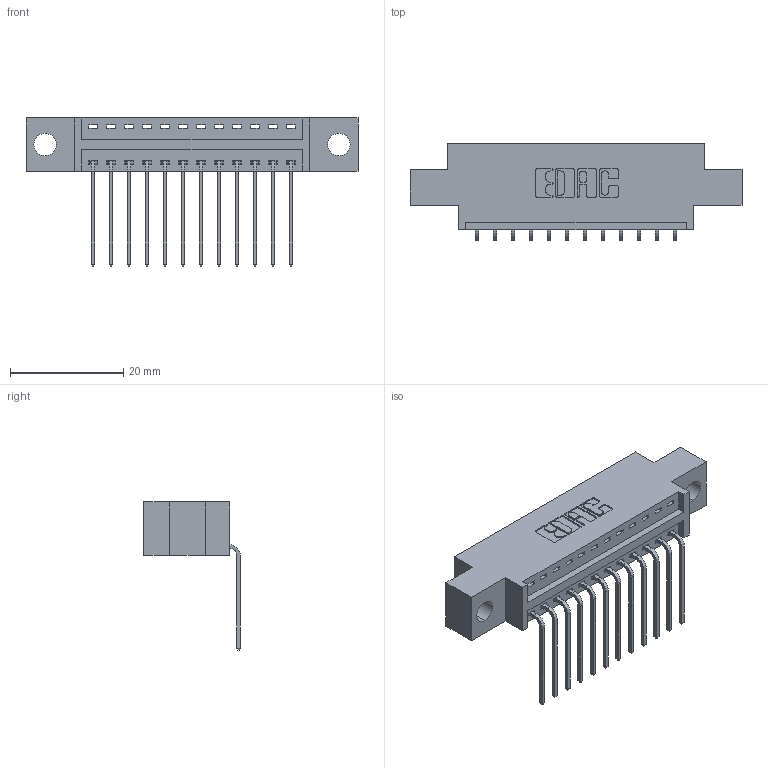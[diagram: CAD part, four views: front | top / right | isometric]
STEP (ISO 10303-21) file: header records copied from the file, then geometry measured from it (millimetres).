
FILE_DESCRIPTION (( 'STEP AP203' ), '1' );
FILE_NAME ('346-012-559-604.STEP', '2022-05-05T03:38:17', ( '' ), ( '' ), 'SwSTEP 2.0', 'SolidWorks 2020', '' );
FILE_SCHEMA (( 'CONFIG_CONTROL_DESIGN' ));
Length unit declared in the file: inch
Products named in the file (3): 345-292-001_558 559 Tail - 1; 346 Part_0.170 Offset - 0.156 Dia-TH; 346-012-559-604
Assembly tree (13 placements, depth 2):
  346-012-559-604
    346 Part_0.170 Offset - 0.156 Dia-TH
    345-292-001_558 559 Tail - 1  x12
Bounding box: 58.67 x 17.08 x 26.16 mm (x, y, z)
Volume: 5189.1 mm3; surface area: 6398.1 mm2
Topology: 13 solids, 13 shells, 860 faces, 2561 edges, 1690 vertices
Faces by surface type: plane 598, cylinder 262
Entity records: 12121 total; most frequent: CARTESIAN_POINT 2098, ORIENTED_EDGE 2042, DIRECTION 1885, EDGE_CURVE 1021, LINE 841, VECTOR 841, VERTEX_POINT 678, AXIS2_PLACEMENT_3D 522
